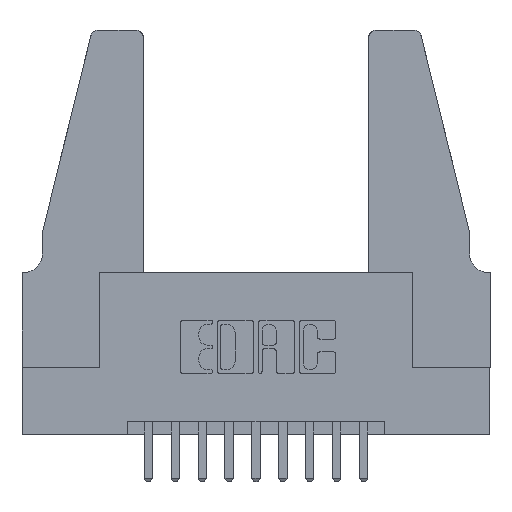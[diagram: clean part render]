
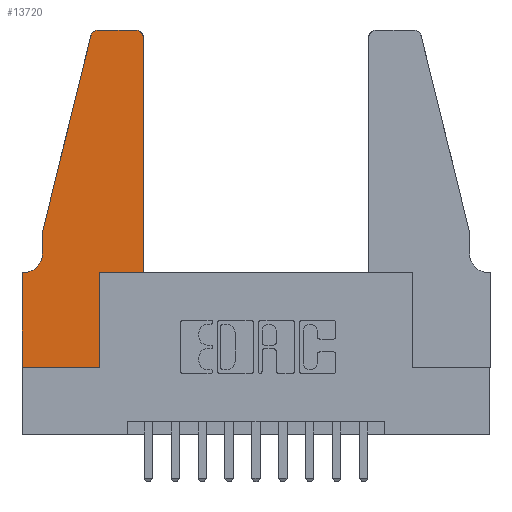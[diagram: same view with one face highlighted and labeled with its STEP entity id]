
A CAD part, top view. The second image highlights one B-rep face of the part: STEP entity #13720.
In plain terms, the highlighted planar face has unit normal (0, 0, 1).
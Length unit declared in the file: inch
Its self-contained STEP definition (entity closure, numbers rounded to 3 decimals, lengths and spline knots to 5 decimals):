
#64 = ORIENTED_EDGE ( 'NONE', *, *, #9478, .T. ) ;
#113 = LINE ( 'NONE', #10795, #3918 ) ;
#387 = AXIS2_PLACEMENT_3D ( 'NONE', #13199, #10437, #7549 ) ;
#512 = CARTESIAN_POINT ( 'NONE',  ( 0.25487, 1.22718, 0.37 ) ) ;
#592 = ORIENTED_EDGE ( 'NONE', *, *, #5206, .T. ) ;
#1003 = ORIENTED_EDGE ( 'NONE', *, *, #8424, .T. ) ;
#1045 = DIRECTION ( 'NONE',  ( 0., -1., 0. ) ) ;
#1222 = VECTOR ( 'NONE', #9314, 39.37008 ) ;
#1387 = VERTEX_POINT ( 'NONE', #12967 ) ;
#1425 = AXIS2_PLACEMENT_3D ( 'NONE', #7916, #2687, #10003 ) ;
#1721 = CARTESIAN_POINT ( 'NONE',  ( 0.0755, 0.35, 0.37 ) ) ;
#1886 = CARTESIAN_POINT ( 'NONE',  ( 0., 0., 0.37 ) ) ;
#2116 = ORIENTED_EDGE ( 'NONE', *, *, #7967, .T. ) ;
#2219 = CARTESIAN_POINT ( 'NONE',  ( 0.0055, 0.42, 0.37 ) ) ;
#2273 = CARTESIAN_POINT ( 'NONE',  ( 0.0755, 0.5, 0.37 ) ) ;
#2288 = EDGE_CURVE ( 'NONE', #3159, #11496, #3086, .T. ) ;
#2299 = DIRECTION ( 'NONE',  ( -0.239, -0.971, 0. ) ) ;
#2351 = CARTESIAN_POINT ( 'NONE',  ( 0.4505, 0.35, 0.37 ) ) ;
#2431 = VERTEX_POINT ( 'NONE', #7621 ) ;
#2531 = CARTESIAN_POINT ( 'NONE',  ( 0., 0.35, 0.37 ) ) ;
#2687 = DIRECTION ( 'NONE',  ( 0., 0., 1. ) ) ;
#3086 = CIRCLE ( 'NONE', #12718, 0.07 ) ;
#3139 = VERTEX_POINT ( 'NONE', #7821 ) ;
#3159 = VERTEX_POINT ( 'NONE', #11756 ) ;
#3563 = CARTESIAN_POINT ( 'NONE',  ( 0.2605, 1.25, 0.37 ) ) ;
#3873 = DIRECTION ( 'NONE',  ( 0., 1., 0. ) ) ;
#3918 = VECTOR ( 'NONE', #11812, 39.37008 ) ;
#4020 = CARTESIAN_POINT ( 'NONE',  ( 0.4205, 1.25, 0.37 ) ) ;
#4068 = VECTOR ( 'NONE', #1045, 39.37008 ) ;
#4162 = EDGE_CURVE ( 'NONE', #2431, #5113, #8653, .T. ) ;
#4440 = CARTESIAN_POINT ( 'NONE',  ( 0.4505, 1.22, 0.37 ) ) ;
#4473 = DIRECTION ( 'NONE',  ( 1., 0., 0. ) ) ;
#4503 = FACE_OUTER_BOUND ( 'NONE', #11651, .T. ) ;
#4836 = LINE ( 'NONE', #1721, #5172 ) ;
#4871 = CARTESIAN_POINT ( 'NONE',  ( 0.0055, 0.35, 0.37 ) ) ;
#5052 = ORIENTED_EDGE ( 'NONE', *, *, #8931, .T. ) ;
#5091 = CARTESIAN_POINT ( 'NONE',  ( 0.0755, 0.5, 0.37 ) ) ;
#5113 = VERTEX_POINT ( 'NONE', #10673 ) ;
#5172 = VECTOR ( 'NONE', #9108, 39.37008 ) ;
#5204 = DIRECTION ( 'NONE',  ( 1., 0., 0. ) ) ;
#5206 = EDGE_CURVE ( 'NONE', #3139, #12974, #6282, .T. ) ;
#5540 = CARTESIAN_POINT ( 'NONE',  ( 0.0755, 0.5, 0.37 ) ) ;
#5565 = ORIENTED_EDGE ( 'NONE', *, *, #4162, .T. ) ;
#6282 = CIRCLE ( 'NONE', #1425, 0.03 ) ;
#6285 = DIRECTION ( 'NONE',  ( -1., 0., 0. ) ) ;
#6348 = AXIS2_PLACEMENT_3D ( 'NONE', #2531, #10870, #4473 ) ;
#6491 = CARTESIAN_POINT ( 'NONE',  ( 0., 0., 0.37 ) ) ;
#6633 = VERTEX_POINT ( 'NONE', #9486 ) ;
#6879 = LINE ( 'NONE', #6491, #4068 ) ;
#6925 = CARTESIAN_POINT ( 'NONE',  ( 0., 0.35, 0.37 ) ) ;
#7056 = VECTOR ( 'NONE', #8709, 39.37008 ) ;
#7265 = VERTEX_POINT ( 'NONE', #4440 ) ;
#7474 = EDGE_CURVE ( 'NONE', #8037, #3139, #13602, .T. ) ;
#7544 = DIRECTION ( 'NONE',  ( 0., 1., 0. ) ) ;
#7549 = DIRECTION ( 'NONE',  ( 1., 0., 0. ) ) ;
#7550 = DIRECTION ( 'NONE',  ( 0., 0., -1. ) ) ;
#7621 = CARTESIAN_POINT ( 'NONE',  ( 0.2865, 0., 0.37 ) ) ;
#7821 = CARTESIAN_POINT ( 'NONE',  ( 0.284, 1.25, 0.37 ) ) ;
#7916 = CARTESIAN_POINT ( 'NONE',  ( 0.284, 1.22, 0.37 ) ) ;
#7967 = EDGE_CURVE ( 'NONE', #12291, #1387, #6879, .T. ) ;
#8037 = VERTEX_POINT ( 'NONE', #4020 ) ;
#8237 = ORIENTED_EDGE ( 'NONE', *, *, #9636, .T. ) ;
#8424 = EDGE_CURVE ( 'NONE', #1387, #2431, #12543, .T. ) ;
#8653 = LINE ( 'NONE', #11158, #9169 ) ;
#8678 = LINE ( 'NONE', #5091, #1222 ) ;
#8709 = DIRECTION ( 'NONE',  ( -1., 0., 0. ) ) ;
#8931 = EDGE_CURVE ( 'NONE', #12974, #13030, #10555, .T. ) ;
#9108 = DIRECTION ( 'NONE',  ( -1., 0., 0. ) ) ;
#9169 = VECTOR ( 'NONE', #3873, 39.37008 ) ;
#9215 = VECTOR ( 'NONE', #5204, 39.37008 ) ;
#9314 = DIRECTION ( 'NONE',  ( 0., -1., 0. ) ) ;
#9478 = EDGE_CURVE ( 'NONE', #13030, #3159, #8678, .T. ) ;
#9486 = CARTESIAN_POINT ( 'NONE',  ( 0.4505, 0.35, 0.37 ) ) ;
#9636 = EDGE_CURVE ( 'NONE', #5113, #6633, #113, .T. ) ;
#9892 = VECTOR ( 'NONE', #2299, 39.37008 ) ;
#9915 = CIRCLE ( 'NONE', #387, 0.03 ) ;
#10003 = DIRECTION ( 'NONE',  ( 1., 0., 0. ) ) ;
#10071 = ORIENTED_EDGE ( 'NONE', *, *, #2288, .T. ) ;
#10274 = ORIENTED_EDGE ( 'NONE', *, *, #13384, .T. ) ;
#10431 = VECTOR ( 'NONE', #7544, 39.37008 ) ;
#10437 = DIRECTION ( 'NONE',  ( 0., 0., 1. ) ) ;
#10555 = LINE ( 'NONE', #5540, #9892 ) ;
#10673 = CARTESIAN_POINT ( 'NONE',  ( 0.2865, 0.35, 0.37 ) ) ;
#10761 = LINE ( 'NONE', #2351, #10431 ) ;
#10795 = CARTESIAN_POINT ( 'NONE',  ( 0.4505, 0.35, 0.37 ) ) ;
#10870 = DIRECTION ( 'NONE',  ( 0., 0., 1. ) ) ;
#10878 = EDGE_CURVE ( 'NONE', #7265, #8037, #9915, .T. ) ;
#11004 = PLANE ( 'NONE',  #6348 ) ;
#11034 = EDGE_CURVE ( 'NONE', #6633, #7265, #10761, .T. ) ;
#11146 = ORIENTED_EDGE ( 'NONE', *, *, #10878, .T. ) ;
#11158 = CARTESIAN_POINT ( 'NONE',  ( 0.2865, 0.35, 0.37 ) ) ;
#11496 = VERTEX_POINT ( 'NONE', #4871 ) ;
#11651 = EDGE_LOOP ( 'NONE', ( #12861, #592, #5052, #64, #10071, #10274, #2116, #1003, #5565, #8237, #12518, #11146 ) ) ;
#11756 = CARTESIAN_POINT ( 'NONE',  ( 0.0755, 0.42, 0.37 ) ) ;
#11812 = DIRECTION ( 'NONE',  ( 1., 0., 0. ) ) ;
#12291 = VERTEX_POINT ( 'NONE', #6925 ) ;
#12518 = ORIENTED_EDGE ( 'NONE', *, *, #11034, .T. ) ;
#12543 = LINE ( 'NONE', #1886, #9215 ) ;
#12718 = AXIS2_PLACEMENT_3D ( 'NONE', #2219, #7550, #6285 ) ;
#12861 = ORIENTED_EDGE ( 'NONE', *, *, #7474, .T. ) ;
#12967 = CARTESIAN_POINT ( 'NONE',  ( 0., 0., 0.37 ) ) ;
#12974 = VERTEX_POINT ( 'NONE', #512 ) ;
#13030 = VERTEX_POINT ( 'NONE', #2273 ) ;
#13199 = CARTESIAN_POINT ( 'NONE',  ( 0.4205, 1.22, 0.37 ) ) ;
#13384 = EDGE_CURVE ( 'NONE', #11496, #12291, #4836, .T. ) ;
#13602 = LINE ( 'NONE', #3563, #7056 ) ;
#13720 = ADVANCED_FACE ( 'NONE', ( #4503 ), #11004, .T. ) ;
